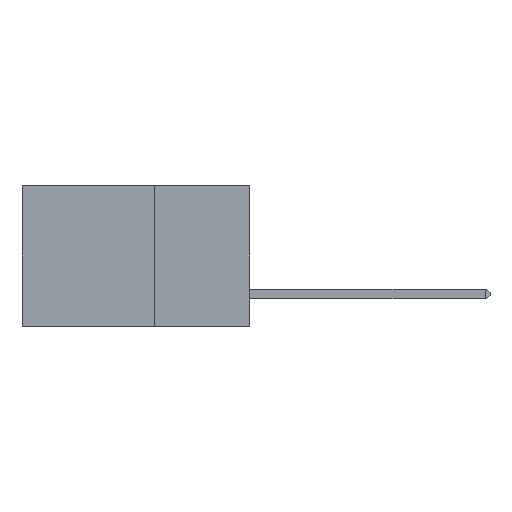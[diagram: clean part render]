
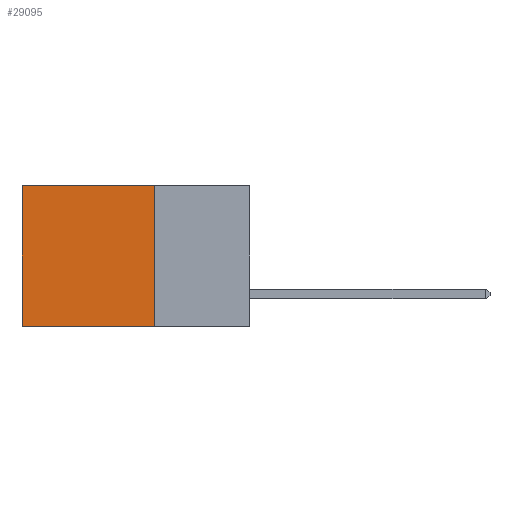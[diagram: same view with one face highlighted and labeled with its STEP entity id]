
A CAD part, left-side view. The second image highlights one B-rep face of the part: STEP entity #29095.
In plain terms, the highlighted planar face has unit normal (-1, 0, 0).
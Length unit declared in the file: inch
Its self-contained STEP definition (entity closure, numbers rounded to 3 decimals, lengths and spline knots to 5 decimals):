
#1349 = DIRECTION ( 'NONE',  ( 1., 0., 0. ) ) ;
#1910 = CARTESIAN_POINT ( 'NONE',  ( 0.2875, 0.25, 0. ) ) ;
#2506 = CARTESIAN_POINT ( 'NONE',  ( 0.2875, 0.6, 0. ) ) ;
#3424 = EDGE_CURVE ( 'NONE', #22647, #8922, #16351, .T. ) ;
#3569 = EDGE_CURVE ( 'NONE', #22412, #8922, #11728, .T. ) ;
#3921 = VECTOR ( 'NONE', #23949, 39.37008 ) ;
#5158 = VECTOR ( 'NONE', #23079, 39.37008 ) ;
#8922 = VERTEX_POINT ( 'NONE', #23222 ) ;
#9472 = EDGE_CURVE ( 'NONE', #16488, #22412, #25210, .T. ) ;
#10278 = ORIENTED_EDGE ( 'NONE', *, *, #9472, .F. ) ;
#10730 = ORIENTED_EDGE ( 'NONE', *, *, #3569, .F. ) ;
#11728 = LINE ( 'NONE', #18165, #5158 ) ;
#12584 = EDGE_LOOP ( 'NONE', ( #25960, #10730, #10278, #13187 ) ) ;
#13187 = ORIENTED_EDGE ( 'NONE', *, *, #30426, .T. ) ;
#13282 = CARTESIAN_POINT ( 'NONE',  ( 0.2875, 0.25, 0. ) ) ;
#14905 = AXIS2_PLACEMENT_3D ( 'NONE', #16049, #1349, #18473 ) ;
#16049 = CARTESIAN_POINT ( 'NONE',  ( 0.2875, 0.25, 0. ) ) ;
#16351 = LINE ( 'NONE', #2506, #29991 ) ;
#16488 = VERTEX_POINT ( 'NONE', #20610 ) ;
#18163 = DIRECTION ( 'NONE',  ( 0., 0., -1. ) ) ;
#18165 = CARTESIAN_POINT ( 'NONE',  ( 0.2875, 0.25, -0.37 ) ) ;
#18473 = DIRECTION ( 'NONE',  ( 0., 0., -1. ) ) ;
#20610 = CARTESIAN_POINT ( 'NONE',  ( 0.2875, 0.25, 0. ) ) ;
#20803 = PLANE ( 'NONE',  #14905 ) ;
#21846 = CARTESIAN_POINT ( 'NONE',  ( 0.2875, 0.25, -0.37 ) ) ;
#22101 = DIRECTION ( 'NONE',  ( 0., 0., -1. ) ) ;
#22412 = VERTEX_POINT ( 'NONE', #21846 ) ;
#22647 = VERTEX_POINT ( 'NONE', #23388 ) ;
#23079 = DIRECTION ( 'NONE',  ( 0., 1., 0. ) ) ;
#23222 = CARTESIAN_POINT ( 'NONE',  ( 0.2875, 0.6, -0.37 ) ) ;
#23388 = CARTESIAN_POINT ( 'NONE',  ( 0.2875, 0.6, 0. ) ) ;
#23949 = DIRECTION ( 'NONE',  ( 0., 1., 0. ) ) ;
#24441 = VECTOR ( 'NONE', #18163, 39.37008 ) ;
#25210 = LINE ( 'NONE', #13282, #24441 ) ;
#25960 = ORIENTED_EDGE ( 'NONE', *, *, #3424, .T. ) ;
#26186 = FACE_OUTER_BOUND ( 'NONE', #12584, .T. ) ;
#29095 = ADVANCED_FACE ( 'NONE', ( #26186 ), #20803, .F. ) ;
#29901 = LINE ( 'NONE', #1910, #3921 ) ;
#29991 = VECTOR ( 'NONE', #22101, 39.37008 ) ;
#30426 = EDGE_CURVE ( 'NONE', #16488, #22647, #29901, .T. ) ;
